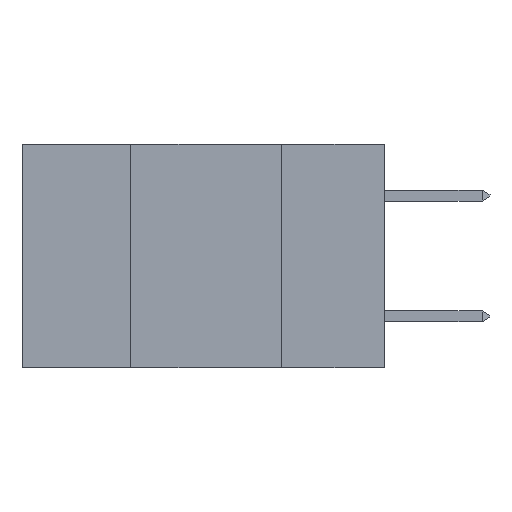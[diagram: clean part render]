
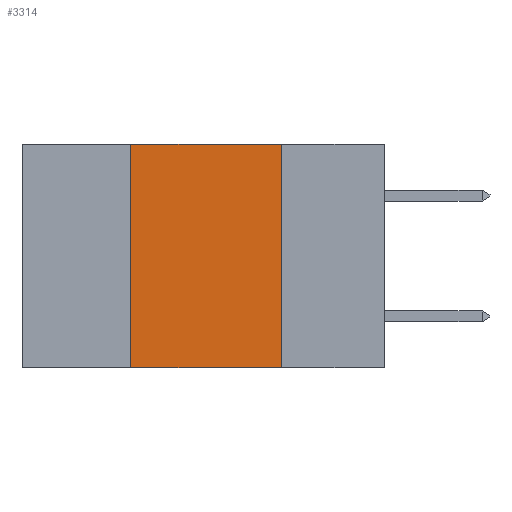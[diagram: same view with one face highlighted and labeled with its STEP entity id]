
A CAD part, left-side view. The second image highlights one B-rep face of the part: STEP entity #3314.
In plain terms, the highlighted planar face has unit normal (-1, 0, 0).
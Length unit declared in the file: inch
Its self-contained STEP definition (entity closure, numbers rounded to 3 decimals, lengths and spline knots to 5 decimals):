
#151 = LINE ( 'NONE', #12473, #7208 ) ;
#173 = ORIENTED_EDGE ( 'NONE', *, *, #10204, .T. ) ;
#422 = DIRECTION ( 'NONE',  ( 1., 0., 0. ) ) ;
#647 = AXIS2_PLACEMENT_3D ( 'NONE', #3806, #422, #16315 ) ;
#648 = VECTOR ( 'NONE', #4173, 39.37008 ) ;
#1186 = DIRECTION ( 'NONE',  ( 0., -1., 0. ) ) ;
#1696 = CARTESIAN_POINT ( 'NONE',  ( 0., 0.42, -0.37 ) ) ;
#2140 = VERTEX_POINT ( 'NONE', #1696 ) ;
#3082 = VERTEX_POINT ( 'NONE', #11865 ) ;
#3257 = PLANE ( 'NONE',  #647 ) ;
#3314 = ADVANCED_FACE ( 'NONE', ( #13540 ), #3257, .F. ) ;
#3523 = CARTESIAN_POINT ( 'NONE',  ( 0., 0.17, 0. ) ) ;
#3806 = CARTESIAN_POINT ( 'NONE',  ( 0., 0.6, 0. ) ) ;
#4173 = DIRECTION ( 'NONE',  ( 0., 0., 1. ) ) ;
#5153 = DIRECTION ( 'NONE',  ( 0., 0., -1. ) ) ;
#5375 = LINE ( 'NONE', #15652, #14710 ) ;
#6098 = CARTESIAN_POINT ( 'NONE',  ( 0., 0.42, 0. ) ) ;
#6161 = EDGE_LOOP ( 'NONE', ( #14797, #11845, #13594, #173 ) ) ;
#6798 = VERTEX_POINT ( 'NONE', #6098 ) ;
#6961 = EDGE_CURVE ( 'NONE', #9216, #3082, #151, .T. ) ;
#7208 = VECTOR ( 'NONE', #5153, 39.37008 ) ;
#9216 = VERTEX_POINT ( 'NONE', #3523 ) ;
#10204 = EDGE_CURVE ( 'NONE', #2140, #3082, #5375, .T. ) ;
#10870 = VECTOR ( 'NONE', #1186, 39.37008 ) ;
#11247 = LINE ( 'NONE', #16152, #10870 ) ;
#11315 = EDGE_CURVE ( 'NONE', #6798, #9216, #11247, .T. ) ;
#11845 = ORIENTED_EDGE ( 'NONE', *, *, #11315, .F. ) ;
#11865 = CARTESIAN_POINT ( 'NONE',  ( 0., 0.17, -0.37 ) ) ;
#12473 = CARTESIAN_POINT ( 'NONE',  ( 0., 0.17, 0. ) ) ;
#12623 = EDGE_CURVE ( 'NONE', #2140, #6798, #14075, .T. ) ;
#12751 = CARTESIAN_POINT ( 'NONE',  ( 0., 0.42, 0. ) ) ;
#13540 = FACE_OUTER_BOUND ( 'NONE', #6161, .T. ) ;
#13594 = ORIENTED_EDGE ( 'NONE', *, *, #12623, .F. ) ;
#14075 = LINE ( 'NONE', #12751, #648 ) ;
#14411 = DIRECTION ( 'NONE',  ( 0., -1., 0. ) ) ;
#14710 = VECTOR ( 'NONE', #14411, 39.37008 ) ;
#14797 = ORIENTED_EDGE ( 'NONE', *, *, #6961, .F. ) ;
#15652 = CARTESIAN_POINT ( 'NONE',  ( 0., 0.6, -0.37 ) ) ;
#16152 = CARTESIAN_POINT ( 'NONE',  ( 0., 0.6, 0. ) ) ;
#16315 = DIRECTION ( 'NONE',  ( 0., 0., -1. ) ) ;
